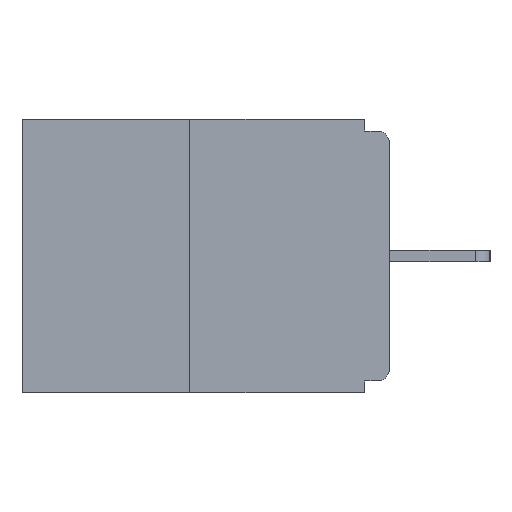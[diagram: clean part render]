
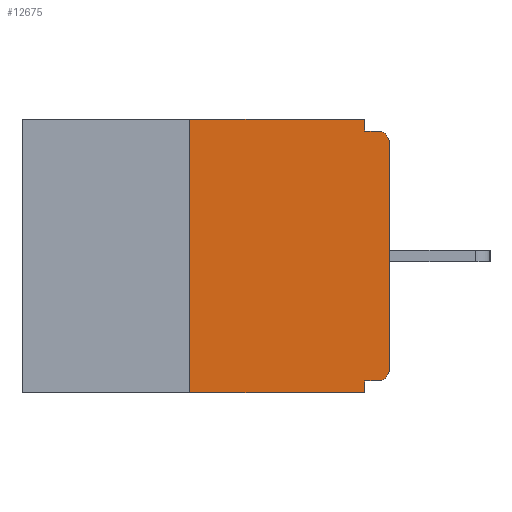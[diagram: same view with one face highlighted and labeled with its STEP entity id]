
A CAD part, left-side view. The second image highlights one B-rep face of the part: STEP entity #12675.
In plain terms, the highlighted planar face has unit normal (-1, 0, 0).
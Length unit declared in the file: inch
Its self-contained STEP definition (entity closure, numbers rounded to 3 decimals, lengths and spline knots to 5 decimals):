
#91 = EDGE_CURVE ( 'NONE', #10515, #7228, #3406, .T. ) ;
#199 = CARTESIAN_POINT ( 'NONE',  ( 0., 0., -0.015 ) ) ;
#1951 = EDGE_CURVE ( 'NONE', #9263, #14541, #4204, .T. ) ;
#2018 = CARTESIAN_POINT ( 'NONE',  ( 0., 0.015, -0.015 ) ) ;
#2028 = DIRECTION ( 'NONE',  ( 0., -1., 0. ) ) ;
#2531 = VECTOR ( 'NONE', #6612, 39.37008 ) ;
#2613 = CARTESIAN_POINT ( 'NONE',  ( 0., 0.25, 0. ) ) ;
#2643 = CARTESIAN_POINT ( 'NONE',  ( 0., 0., -0.328 ) ) ;
#2671 = CARTESIAN_POINT ( 'NONE',  ( 0., 0.25, 0. ) ) ;
#2744 = CARTESIAN_POINT ( 'NONE',  ( 0., 0.46, 0. ) ) ;
#3295 = ORIENTED_EDGE ( 'NONE', *, *, #5216, .F. ) ;
#3406 = LINE ( 'NONE', #4758, #8412 ) ;
#3427 = CARTESIAN_POINT ( 'NONE',  ( 0., 0.031, 0. ) ) ;
#3613 = CARTESIAN_POINT ( 'NONE',  ( 0., 0.031, -0.015 ) ) ;
#3959 = ORIENTED_EDGE ( 'NONE', *, *, #8112, .T. ) ;
#4204 = CIRCLE ( 'NONE', #16293, 0.015 ) ;
#4267 = AXIS2_PLACEMENT_3D ( 'NONE', #9677, #21980, #9458 ) ;
#4352 = PLANE ( 'NONE',  #9613 ) ;
#4396 = CARTESIAN_POINT ( 'NONE',  ( 0., 0., -0.03 ) ) ;
#4608 = VECTOR ( 'NONE', #17286, 39.37008 ) ;
#4679 = LINE ( 'NONE', #8240, #16841 ) ;
#4758 = CARTESIAN_POINT ( 'NONE',  ( 0., 0.46, -0.343 ) ) ;
#5031 = EDGE_CURVE ( 'NONE', #17342, #15763, #17049, .T. ) ;
#5216 = EDGE_CURVE ( 'NONE', #15763, #7228, #20885, .T. ) ;
#6347 = EDGE_CURVE ( 'NONE', #10515, #20344, #7710, .T. ) ;
#6453 = CARTESIAN_POINT ( 'NONE',  ( 0., 0.031, 0. ) ) ;
#6488 = EDGE_CURVE ( 'NONE', #8270, #14507, #19140, .T. ) ;
#6612 = DIRECTION ( 'NONE',  ( 0., 0., 1. ) ) ;
#6740 = CARTESIAN_POINT ( 'NONE',  ( 0., 0., -0.313 ) ) ;
#6884 = DIRECTION ( 'NONE',  ( 0., 0., -1. ) ) ;
#7214 = CARTESIAN_POINT ( 'NONE',  ( 0., 0.015, -0.328 ) ) ;
#7228 = VERTEX_POINT ( 'NONE', #12206 ) ;
#7710 = LINE ( 'NONE', #2671, #2531 ) ;
#7892 = FACE_OUTER_BOUND ( 'NONE', #16452, .T. ) ;
#8112 = EDGE_CURVE ( 'NONE', #11221, #9263, #4679, .T. ) ;
#8240 = CARTESIAN_POINT ( 'NONE',  ( 0., 0., 0. ) ) ;
#8270 = VERTEX_POINT ( 'NONE', #6453 ) ;
#8412 = VECTOR ( 'NONE', #17899, 39.37008 ) ;
#8705 = CARTESIAN_POINT ( 'NONE',  ( 0., 0.031, -0.343 ) ) ;
#8899 = LINE ( 'NONE', #199, #9765 ) ;
#9248 = ORIENTED_EDGE ( 'NONE', *, *, #91, .T. ) ;
#9263 = VERTEX_POINT ( 'NONE', #4396 ) ;
#9458 = DIRECTION ( 'NONE',  ( 0., 0., -1. ) ) ;
#9613 = AXIS2_PLACEMENT_3D ( 'NONE', #2744, #19969, #9853 ) ;
#9677 = CARTESIAN_POINT ( 'NONE',  ( 0., 0.015, -0.313 ) ) ;
#9765 = VECTOR ( 'NONE', #2028, 39.37008 ) ;
#9853 = DIRECTION ( 'NONE',  ( 0., 0., -1. ) ) ;
#10238 = LINE ( 'NONE', #20587, #18927 ) ;
#10282 = ORIENTED_EDGE ( 'NONE', *, *, #18026, .F. ) ;
#10515 = VERTEX_POINT ( 'NONE', #14751 ) ;
#11221 = VERTEX_POINT ( 'NONE', #6740 ) ;
#11695 = DIRECTION ( 'NONE',  ( 0., 0., 1. ) ) ;
#12206 = CARTESIAN_POINT ( 'NONE',  ( 0., 0.031, -0.343 ) ) ;
#12256 = DIRECTION ( 'NONE',  ( 0., 0., -1. ) ) ;
#12311 = ORIENTED_EDGE ( 'NONE', *, *, #1951, .T. ) ;
#12675 = ADVANCED_FACE ( 'NONE', ( #7892 ), #4352, .F. ) ;
#13566 = ORIENTED_EDGE ( 'NONE', *, *, #5031, .F. ) ;
#14050 = CARTESIAN_POINT ( 'NONE',  ( 0., 0.031, -0.328 ) ) ;
#14507 = VERTEX_POINT ( 'NONE', #3613 ) ;
#14541 = VERTEX_POINT ( 'NONE', #2018 ) ;
#14751 = CARTESIAN_POINT ( 'NONE',  ( 0., 0.25, -0.343 ) ) ;
#15717 = CARTESIAN_POINT ( 'NONE',  ( 0., 0.015, -0.03 ) ) ;
#15763 = VERTEX_POINT ( 'NONE', #14050 ) ;
#16293 = AXIS2_PLACEMENT_3D ( 'NONE', #15717, #21271, #6884 ) ;
#16452 = EDGE_LOOP ( 'NONE', ( #10282, #20257, #9248, #3295, #13566, #18295, #3959, #12311, #16892, #19071 ) ) ;
#16841 = VECTOR ( 'NONE', #11695, 39.37008 ) ;
#16892 = ORIENTED_EDGE ( 'NONE', *, *, #20648, .F. ) ;
#17049 = LINE ( 'NONE', #2643, #20425 ) ;
#17067 = CIRCLE ( 'NONE', #4267, 0.015 ) ;
#17286 = DIRECTION ( 'NONE',  ( 0., 0., -1. ) ) ;
#17342 = VERTEX_POINT ( 'NONE', #7214 ) ;
#17885 = EDGE_CURVE ( 'NONE', #17342, #11221, #17067, .T. ) ;
#17899 = DIRECTION ( 'NONE',  ( 0., -1., 0. ) ) ;
#18026 = EDGE_CURVE ( 'NONE', #20344, #8270, #10238, .T. ) ;
#18295 = ORIENTED_EDGE ( 'NONE', *, *, #17885, .T. ) ;
#18927 = VECTOR ( 'NONE', #18967, 39.37008 ) ;
#18967 = DIRECTION ( 'NONE',  ( 0., -1., 0. ) ) ;
#19071 = ORIENTED_EDGE ( 'NONE', *, *, #6488, .F. ) ;
#19140 = LINE ( 'NONE', #3427, #4608 ) ;
#19969 = DIRECTION ( 'NONE',  ( 1., 0., 0. ) ) ;
#20257 = ORIENTED_EDGE ( 'NONE', *, *, #6347, .F. ) ;
#20344 = VERTEX_POINT ( 'NONE', #2613 ) ;
#20425 = VECTOR ( 'NONE', #22037, 39.37008 ) ;
#20587 = CARTESIAN_POINT ( 'NONE',  ( 0., 0.46, 0. ) ) ;
#20648 = EDGE_CURVE ( 'NONE', #14507, #14541, #8899, .T. ) ;
#20885 = LINE ( 'NONE', #8705, #21576 ) ;
#21271 = DIRECTION ( 'NONE',  ( -1., 0., 0. ) ) ;
#21576 = VECTOR ( 'NONE', #12256, 39.37008 ) ;
#21980 = DIRECTION ( 'NONE',  ( -1., 0., 0. ) ) ;
#22037 = DIRECTION ( 'NONE',  ( 0., 1., 0. ) ) ;
